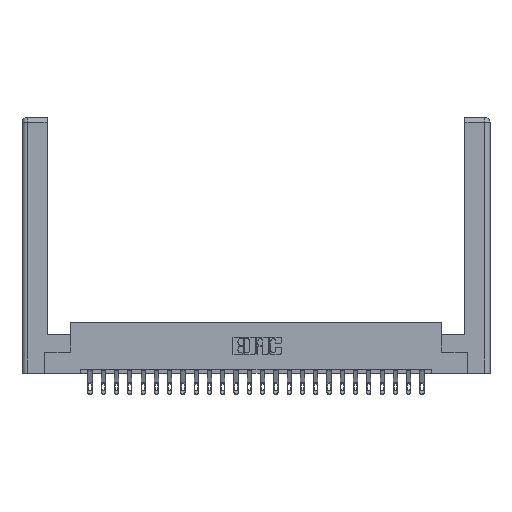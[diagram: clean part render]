
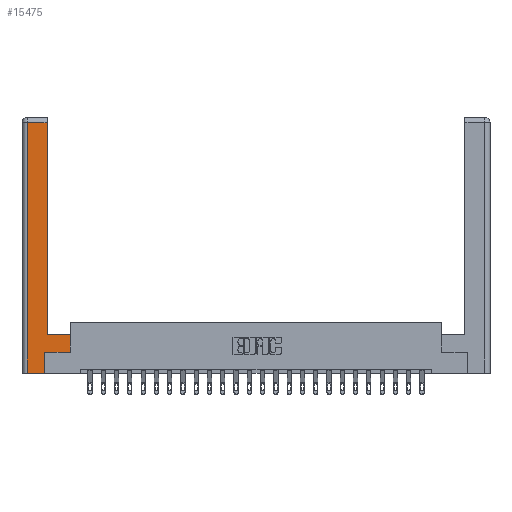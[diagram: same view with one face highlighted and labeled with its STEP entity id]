
A CAD part, top view. The second image highlights one B-rep face of the part: STEP entity #15475.
In plain terms, the highlighted planar face has unit normal (0, 0, 1).
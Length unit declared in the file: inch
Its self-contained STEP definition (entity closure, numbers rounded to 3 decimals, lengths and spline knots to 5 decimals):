
#121 = DIRECTION ( 'NONE',  ( 0., 1., 0. ) ) ;
#156 = LINE ( 'NONE', #15805, #20902 ) ;
#594 = CARTESIAN_POINT ( 'NONE',  ( 0.565, 0.245, 0. ) ) ;
#858 = DIRECTION ( 'NONE',  ( 1., 0., 0. ) ) ;
#878 = VECTOR ( 'NONE', #858, 39.37008 ) ;
#1149 = EDGE_CURVE ( 'NONE', #3343, #20057, #11161, .T. ) ;
#1535 = DIRECTION ( 'NONE',  ( -1., 0., 0. ) ) ;
#1591 = DIRECTION ( 'NONE',  ( 0., 1., 0. ) ) ;
#1726 = VERTEX_POINT ( 'NONE', #21999 ) ;
#2596 = VECTOR ( 'NONE', #19783, 39.37008 ) ;
#2873 = AXIS2_PLACEMENT_3D ( 'NONE', #20740, #20583, #8747 ) ;
#3179 = CARTESIAN_POINT ( 'NONE',  ( 0.295, 2.94, 0. ) ) ;
#3343 = VERTEX_POINT ( 'NONE', #11466 ) ;
#3660 = CARTESIAN_POINT ( 'NONE',  ( 0.295, 3., 0. ) ) ;
#4499 = LINE ( 'NONE', #18806, #9609 ) ;
#4822 = PLANE ( 'NONE',  #2873 ) ;
#5557 = ORIENTED_EDGE ( 'NONE', *, *, #15306, .T. ) ;
#6885 = CARTESIAN_POINT ( 'NONE',  ( 0.265, 0.245, 0. ) ) ;
#8747 = DIRECTION ( 'NONE',  ( -1., 0., 0. ) ) ;
#9609 = VECTOR ( 'NONE', #24645, 39.37008 ) ;
#9910 = VECTOR ( 'NONE', #24698, 39.37008 ) ;
#10066 = ORIENTED_EDGE ( 'NONE', *, *, #17609, .T. ) ;
#10684 = EDGE_LOOP ( 'NONE', ( #19629, #19689, #24914, #13952, #5557, #21566, #10066, #19268 ) ) ;
#10750 = CARTESIAN_POINT ( 'NONE',  ( 0.565, 0.45, 0. ) ) ;
#11160 = LINE ( 'NONE', #17121, #15468 ) ;
#11161 = LINE ( 'NONE', #3660, #23396 ) ;
#11466 = CARTESIAN_POINT ( 'NONE',  ( 0.295, 0.45, 0. ) ) ;
#13952 = ORIENTED_EDGE ( 'NONE', *, *, #19649, .T. ) ;
#14563 = EDGE_CURVE ( 'NONE', #23874, #15151, #4499, .T. ) ;
#14822 = VECTOR ( 'NONE', #1591, 39.37008 ) ;
#15151 = VERTEX_POINT ( 'NONE', #17443 ) ;
#15306 = EDGE_CURVE ( 'NONE', #17557, #20923, #156, .T. ) ;
#15468 = VECTOR ( 'NONE', #1535, 39.37008 ) ;
#15475 = ADVANCED_FACE ( 'NONE', ( #18507 ), #4822, .F. ) ;
#15781 = CARTESIAN_POINT ( 'NONE',  ( 0.0615, 2.94, 0. ) ) ;
#15805 = CARTESIAN_POINT ( 'NONE',  ( 0.265, 0.245, 0. ) ) ;
#16431 = LINE ( 'NONE', #594, #878 ) ;
#17094 = EDGE_CURVE ( 'NONE', #20923, #23241, #16431, .T. ) ;
#17121 = CARTESIAN_POINT ( 'NONE',  ( 0.295, 0.45, 0. ) ) ;
#17443 = CARTESIAN_POINT ( 'NONE',  ( 0.0615, 0., 0. ) ) ;
#17557 = VERTEX_POINT ( 'NONE', #20363 ) ;
#17609 = EDGE_CURVE ( 'NONE', #23241, #1726, #23674, .T. ) ;
#18175 = LINE ( 'NONE', #21618, #2596 ) ;
#18507 = FACE_OUTER_BOUND ( 'NONE', #10684, .T. ) ;
#18712 = CARTESIAN_POINT ( 'NONE',  ( 0.0615, 2.94, 0. ) ) ;
#18806 = CARTESIAN_POINT ( 'NONE',  ( 0.0615, 0., 0. ) ) ;
#19263 = DIRECTION ( 'NONE',  ( 0., 1., 0. ) ) ;
#19268 = ORIENTED_EDGE ( 'NONE', *, *, #23927, .T. ) ;
#19629 = ORIENTED_EDGE ( 'NONE', *, *, #1149, .T. ) ;
#19649 = EDGE_CURVE ( 'NONE', #15151, #17557, #18175, .T. ) ;
#19689 = ORIENTED_EDGE ( 'NONE', *, *, #24412, .T. ) ;
#19783 = DIRECTION ( 'NONE',  ( 1., 0., 0. ) ) ;
#20057 = VERTEX_POINT ( 'NONE', #3179 ) ;
#20363 = CARTESIAN_POINT ( 'NONE',  ( 0.265, 0., 0. ) ) ;
#20583 = DIRECTION ( 'NONE',  ( 0., 0., -1. ) ) ;
#20740 = CARTESIAN_POINT ( 'NONE',  ( 0., 0., 0. ) ) ;
#20902 = VECTOR ( 'NONE', #121, 39.37008 ) ;
#20923 = VERTEX_POINT ( 'NONE', #6885 ) ;
#21566 = ORIENTED_EDGE ( 'NONE', *, *, #17094, .T. ) ;
#21618 = CARTESIAN_POINT ( 'NONE',  ( 0.265, 0., 0. ) ) ;
#21999 = CARTESIAN_POINT ( 'NONE',  ( 0.565, 0.45, 0. ) ) ;
#22475 = LINE ( 'NONE', #18712, #9910 ) ;
#23241 = VERTEX_POINT ( 'NONE', #24719 ) ;
#23396 = VECTOR ( 'NONE', #19263, 39.37008 ) ;
#23674 = LINE ( 'NONE', #10750, #14822 ) ;
#23874 = VERTEX_POINT ( 'NONE', #15781 ) ;
#23927 = EDGE_CURVE ( 'NONE', #1726, #3343, #11160, .T. ) ;
#24412 = EDGE_CURVE ( 'NONE', #20057, #23874, #22475, .T. ) ;
#24645 = DIRECTION ( 'NONE',  ( 0., -1., 0. ) ) ;
#24698 = DIRECTION ( 'NONE',  ( -1., 0., 0. ) ) ;
#24719 = CARTESIAN_POINT ( 'NONE',  ( 0.565, 0.245, 0. ) ) ;
#24914 = ORIENTED_EDGE ( 'NONE', *, *, #14563, .T. ) ;
